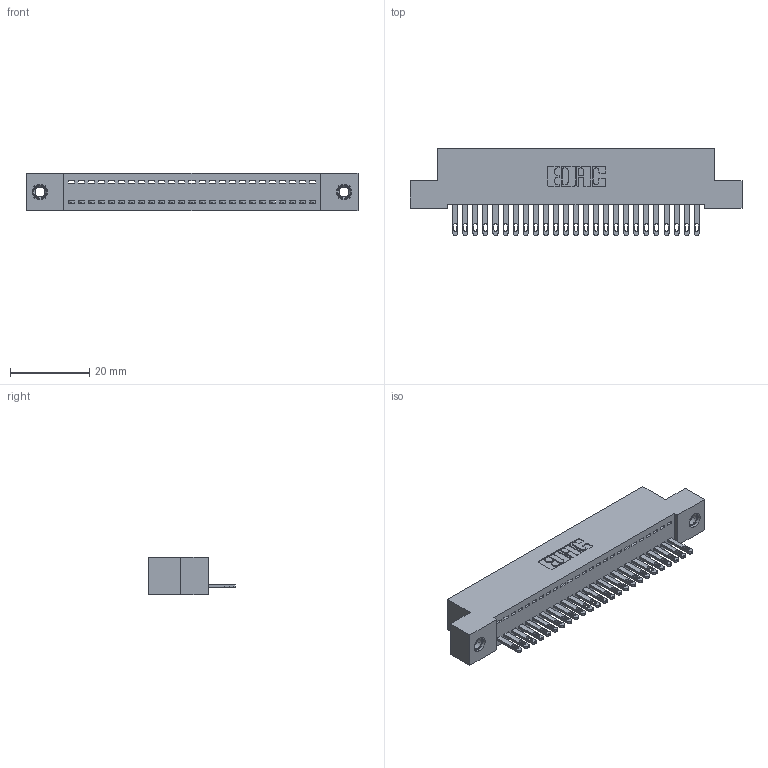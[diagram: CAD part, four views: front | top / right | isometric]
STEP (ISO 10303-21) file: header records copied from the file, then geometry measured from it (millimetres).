
FILE_DESCRIPTION (( 'STEP AP203' ), '1' );
FILE_NAME ('892-025-500-107.STEP', '2020-09-21T14:32:08', ( '' ), ( '' ), 'SwSTEP 2.0', 'SolidWorks 2020', '' );
FILE_SCHEMA (( 'CONFIG_CONTROL_DESIGN' ));
Length unit declared in the file: inch
Products named in the file (4): 345-292-001_345-293-100; 842 Part_TI; 345-250-001_345-250-005-103; 892-025-500-107
Assembly tree (28 placements, depth 2):
  892-025-500-107
    842 Part_TI
    345-292-001_345-293-100  x25
    345-250-001_345-250-005-103  x2
Bounding box: 83.82 x 21.85 x 9.4 mm (x, y, z)
Volume: 7289.5 mm3; surface area: 10468.3 mm2
Topology: 28 solids, 28 shells, 1520 faces, 4635 edges, 3082 vertices
Faces by surface type: plane 998, cylinder 506, cone 12, torus 4
Entity records: 18466 total; most frequent: CARTESIAN_POINT 3168, ORIENTED_EDGE 3122, DIRECTION 2741, EDGE_CURVE 1561, VECTOR 1409, LINE 1409, VERTEX_POINT 1036, AXIS2_PLACEMENT_3D 666
